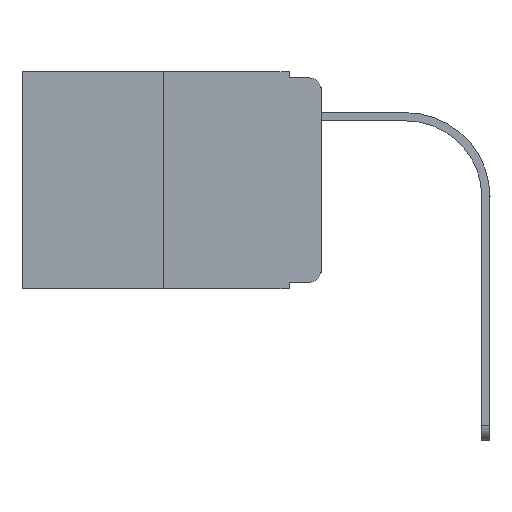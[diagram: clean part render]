
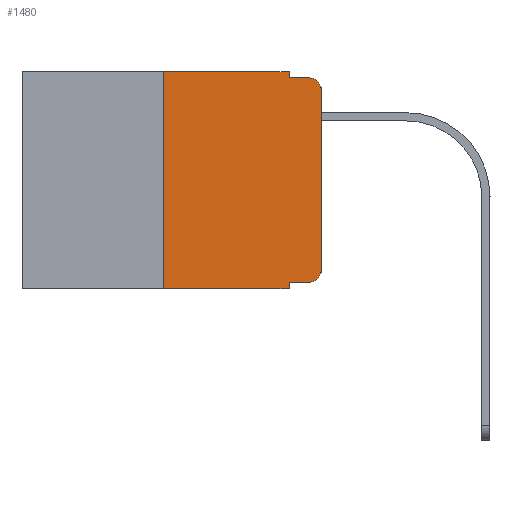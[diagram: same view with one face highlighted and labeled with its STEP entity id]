
A CAD part, left-side view. The second image highlights one B-rep face of the part: STEP entity #1480.
In plain terms, the highlighted planar face has unit normal (-1, 0, 0).
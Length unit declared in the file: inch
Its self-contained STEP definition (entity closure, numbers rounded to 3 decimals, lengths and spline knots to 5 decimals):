
#14 = CARTESIAN_POINT ( 'NONE',  ( 0., 0.051, -0.01 ) ) ;
#25 = DIRECTION ( 'NONE',  ( 0., 0., 1. ) ) ;
#323 = ORIENTED_EDGE ( 'NONE', *, *, #7428, .F. ) ;
#339 = DIRECTION ( 'NONE',  ( 0., -1., 0. ) ) ;
#627 = DIRECTION ( 'NONE',  ( 0., 0., -1. ) ) ;
#898 = VERTEX_POINT ( 'NONE', #2115 ) ;
#1061 = LINE ( 'NONE', #14, #1770 ) ;
#1101 = CIRCLE ( 'NONE', #4909, 0.02 ) ;
#1207 = ORIENTED_EDGE ( 'NONE', *, *, #10931, .F. ) ;
#1239 = CARTESIAN_POINT ( 'NONE',  ( 0., 0.473, 0. ) ) ;
#1283 = CARTESIAN_POINT ( 'NONE',  ( 0., 0., -0.03 ) ) ;
#1423 = AXIS2_PLACEMENT_3D ( 'NONE', #1239, #9438, #5340 ) ;
#1480 = ADVANCED_FACE ( 'NONE', ( #12540 ), #5400, .F. ) ;
#1619 = CARTESIAN_POINT ( 'NONE',  ( 0., 0.051, -0.01 ) ) ;
#1621 = LINE ( 'NONE', #2420, #7881 ) ;
#1770 = VECTOR ( 'NONE', #5093, 39.37008 ) ;
#1813 = CARTESIAN_POINT ( 'NONE',  ( 0., 0., 0. ) ) ;
#2001 = LINE ( 'NONE', #10009, #7382 ) ;
#2115 = CARTESIAN_POINT ( 'NONE',  ( 0., 0.25, -0.343 ) ) ;
#2179 = ORIENTED_EDGE ( 'NONE', *, *, #6804, .F. ) ;
#2420 = CARTESIAN_POINT ( 'NONE',  ( 0., 0.051, 0. ) ) ;
#2748 = VERTEX_POINT ( 'NONE', #11163 ) ;
#2989 = EDGE_CURVE ( 'NONE', #9866, #5019, #5917, .T. ) ;
#3110 = EDGE_CURVE ( 'NONE', #898, #5019, #8040, .T. ) ;
#3254 = CARTESIAN_POINT ( 'NONE',  ( 0., 0.051, 0. ) ) ;
#3769 = CARTESIAN_POINT ( 'NONE',  ( 0., 0.02, -0.333 ) ) ;
#3802 = EDGE_CURVE ( 'NONE', #9927, #2748, #11616, .T. ) ;
#3894 = CARTESIAN_POINT ( 'NONE',  ( 0., 0.02, -0.313 ) ) ;
#4563 = CARTESIAN_POINT ( 'NONE',  ( 0., 0.25, 0. ) ) ;
#4657 = VERTEX_POINT ( 'NONE', #12525 ) ;
#4748 = CARTESIAN_POINT ( 'NONE',  ( 0., 0.051, 0. ) ) ;
#4850 = AXIS2_PLACEMENT_3D ( 'NONE', #5999, #11969, #8780 ) ;
#4909 = AXIS2_PLACEMENT_3D ( 'NONE', #3894, #9905, #11967 ) ;
#5019 = VERTEX_POINT ( 'NONE', #12511 ) ;
#5093 = DIRECTION ( 'NONE',  ( 0., -1., 0. ) ) ;
#5340 = DIRECTION ( 'NONE',  ( 0., 0., -1. ) ) ;
#5400 = PLANE ( 'NONE',  #1423 ) ;
#5917 = LINE ( 'NONE', #4748, #11413 ) ;
#5999 = CARTESIAN_POINT ( 'NONE',  ( 0., 0.02, -0.03 ) ) ;
#6197 = CARTESIAN_POINT ( 'NONE',  ( 0., 0.051, -0.333 ) ) ;
#6548 = EDGE_LOOP ( 'NONE', ( #8643, #8942, #323, #2179, #11648, #1207, #7460, #12287, #11035, #9484 ) ) ;
#6786 = DIRECTION ( 'NONE',  ( 0., 0., -1. ) ) ;
#6804 = EDGE_CURVE ( 'NONE', #11645, #11395, #1621, .T. ) ;
#7049 = CARTESIAN_POINT ( 'NONE',  ( 0., 0.051, -0.333 ) ) ;
#7358 = CARTESIAN_POINT ( 'NONE',  ( 0., 0.25, 0. ) ) ;
#7382 = VECTOR ( 'NONE', #10126, 39.37008 ) ;
#7428 = EDGE_CURVE ( 'NONE', #11395, #2748, #1061, .T. ) ;
#7460 = ORIENTED_EDGE ( 'NONE', *, *, #3110, .T. ) ;
#7481 = DIRECTION ( 'NONE',  ( 0., 0., 1. ) ) ;
#7617 = VECTOR ( 'NONE', #7481, 39.37008 ) ;
#7669 = VECTOR ( 'NONE', #9170, 39.37008 ) ;
#7742 = VERTEX_POINT ( 'NONE', #3769 ) ;
#7881 = VECTOR ( 'NONE', #627, 39.37008 ) ;
#8018 = LINE ( 'NONE', #1813, #11833 ) ;
#8040 = LINE ( 'NONE', #11092, #10967 ) ;
#8397 = VERTEX_POINT ( 'NONE', #7358 ) ;
#8643 = ORIENTED_EDGE ( 'NONE', *, *, #10288, .T. ) ;
#8780 = DIRECTION ( 'NONE',  ( 0., 0., -1. ) ) ;
#8942 = ORIENTED_EDGE ( 'NONE', *, *, #3802, .T. ) ;
#9170 = DIRECTION ( 'NONE',  ( 0., -1., 0. ) ) ;
#9438 = DIRECTION ( 'NONE',  ( 1., 0., 0. ) ) ;
#9484 = ORIENTED_EDGE ( 'NONE', *, *, #12446, .T. ) ;
#9511 = LINE ( 'NONE', #4563, #7617 ) ;
#9866 = VERTEX_POINT ( 'NONE', #7049 ) ;
#9905 = DIRECTION ( 'NONE',  ( -1., 0., 0. ) ) ;
#9927 = VERTEX_POINT ( 'NONE', #1283 ) ;
#10009 = CARTESIAN_POINT ( 'NONE',  ( 0., 0.473, 0. ) ) ;
#10095 = LINE ( 'NONE', #6197, #7669 ) ;
#10126 = DIRECTION ( 'NONE',  ( 0., -1., 0. ) ) ;
#10212 = EDGE_CURVE ( 'NONE', #8397, #11645, #2001, .T. ) ;
#10288 = EDGE_CURVE ( 'NONE', #4657, #9927, #8018, .T. ) ;
#10931 = EDGE_CURVE ( 'NONE', #898, #8397, #9511, .T. ) ;
#10967 = VECTOR ( 'NONE', #339, 39.37008 ) ;
#11035 = ORIENTED_EDGE ( 'NONE', *, *, #12506, .T. ) ;
#11092 = CARTESIAN_POINT ( 'NONE',  ( 0., 0.473, -0.343 ) ) ;
#11163 = CARTESIAN_POINT ( 'NONE',  ( 0., 0.02, -0.01 ) ) ;
#11395 = VERTEX_POINT ( 'NONE', #1619 ) ;
#11413 = VECTOR ( 'NONE', #6786, 39.37008 ) ;
#11616 = CIRCLE ( 'NONE', #4850, 0.02 ) ;
#11645 = VERTEX_POINT ( 'NONE', #3254 ) ;
#11648 = ORIENTED_EDGE ( 'NONE', *, *, #10212, .F. ) ;
#11833 = VECTOR ( 'NONE', #25, 39.37008 ) ;
#11967 = DIRECTION ( 'NONE',  ( 0., 0., -1. ) ) ;
#11969 = DIRECTION ( 'NONE',  ( -1., 0., 0. ) ) ;
#12287 = ORIENTED_EDGE ( 'NONE', *, *, #2989, .F. ) ;
#12446 = EDGE_CURVE ( 'NONE', #7742, #4657, #1101, .T. ) ;
#12506 = EDGE_CURVE ( 'NONE', #9866, #7742, #10095, .T. ) ;
#12511 = CARTESIAN_POINT ( 'NONE',  ( 0., 0.051, -0.343 ) ) ;
#12525 = CARTESIAN_POINT ( 'NONE',  ( 0., 0., -0.313 ) ) ;
#12540 = FACE_OUTER_BOUND ( 'NONE', #6548, .T. ) ;
